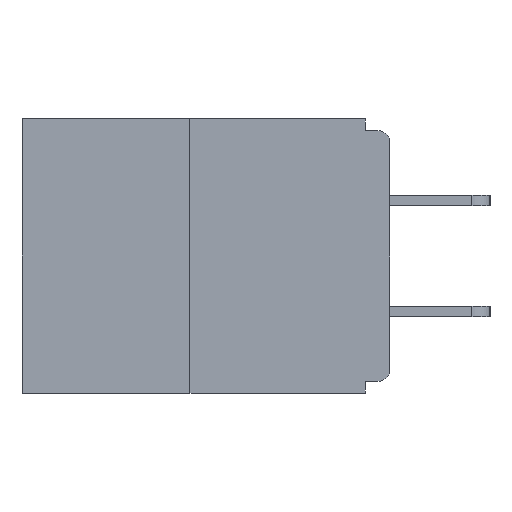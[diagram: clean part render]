
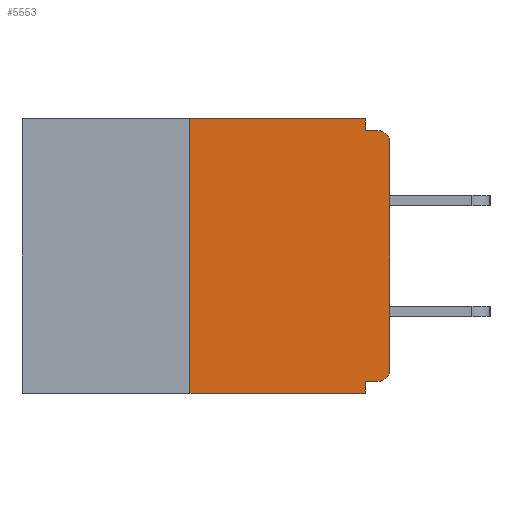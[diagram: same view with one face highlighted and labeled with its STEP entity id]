
A CAD part, left-side view. The second image highlights one B-rep face of the part: STEP entity #5553.
In plain terms, the highlighted planar face has unit normal (-1, 0, 0).
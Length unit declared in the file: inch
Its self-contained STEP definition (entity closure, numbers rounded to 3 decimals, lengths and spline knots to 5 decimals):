
#9 = CARTESIAN_POINT ( 'NONE',  ( 0., 0.031, -0.343 ) ) ;
#730 = VERTEX_POINT ( 'NONE', #9 ) ;
#958 = VECTOR ( 'NONE', #14906, 39.37008 ) ;
#1093 = CARTESIAN_POINT ( 'NONE',  ( 0., 0.015, -0.313 ) ) ;
#1109 = DIRECTION ( 'NONE',  ( 0., -1., 0. ) ) ;
#1291 = VERTEX_POINT ( 'NONE', #16873 ) ;
#1511 = ORIENTED_EDGE ( 'NONE', *, *, #15833, .F. ) ;
#1724 = CARTESIAN_POINT ( 'NONE',  ( 0., 0., -0.03 ) ) ;
#1738 = DIRECTION ( 'NONE',  ( 0., 0., 1. ) ) ;
#2179 = DIRECTION ( 'NONE',  ( 0., 0., -1. ) ) ;
#2210 = VERTEX_POINT ( 'NONE', #12790 ) ;
#2309 = ORIENTED_EDGE ( 'NONE', *, *, #11616, .T. ) ;
#2438 = VERTEX_POINT ( 'NONE', #8670 ) ;
#2523 = LINE ( 'NONE', #8160, #10236 ) ;
#2908 = VERTEX_POINT ( 'NONE', #13664 ) ;
#3392 = EDGE_CURVE ( 'NONE', #2210, #2438, #9552, .T. ) ;
#3741 = ORIENTED_EDGE ( 'NONE', *, *, #15880, .F. ) ;
#3826 = CARTESIAN_POINT ( 'NONE',  ( 0., 0.46, 0. ) ) ;
#4283 = VECTOR ( 'NONE', #13212, 39.37008 ) ;
#4458 = VECTOR ( 'NONE', #1109, 39.37008 ) ;
#4940 = DIRECTION ( 'NONE',  ( -1., 0., 0. ) ) ;
#5096 = EDGE_CURVE ( 'NONE', #2210, #730, #12854, .T. ) ;
#5266 = FACE_OUTER_BOUND ( 'NONE', #16111, .T. ) ;
#5387 = ORIENTED_EDGE ( 'NONE', *, *, #9527, .F. ) ;
#5483 = DIRECTION ( 'NONE',  ( -1., 0., 0. ) ) ;
#5553 = ADVANCED_FACE ( 'NONE', ( #5266 ), #6239, .F. ) ;
#5596 = CARTESIAN_POINT ( 'NONE',  ( 0., 0., -0.313 ) ) ;
#5627 = CARTESIAN_POINT ( 'NONE',  ( 0., 0.015, -0.328 ) ) ;
#5734 = DIRECTION ( 'NONE',  ( 0., 0., -1. ) ) ;
#6239 = PLANE ( 'NONE',  #13242 ) ;
#6266 = ORIENTED_EDGE ( 'NONE', *, *, #5096, .T. ) ;
#6749 = EDGE_CURVE ( 'NONE', #7944, #10308, #14584, .T. ) ;
#6759 = CARTESIAN_POINT ( 'NONE',  ( 0., 0.031, -0.343 ) ) ;
#6808 = CARTESIAN_POINT ( 'NONE',  ( 0., 0., 0. ) ) ;
#7686 = DIRECTION ( 'NONE',  ( 0., 0., -1. ) ) ;
#7709 = EDGE_CURVE ( 'NONE', #2438, #2908, #12510, .T. ) ;
#7856 = ORIENTED_EDGE ( 'NONE', *, *, #15034, .F. ) ;
#7944 = VERTEX_POINT ( 'NONE', #5627 ) ;
#8093 = LINE ( 'NONE', #6808, #4283 ) ;
#8160 = CARTESIAN_POINT ( 'NONE',  ( 0., 0., -0.015 ) ) ;
#8259 = VERTEX_POINT ( 'NONE', #15384 ) ;
#8479 = VERTEX_POINT ( 'NONE', #1724 ) ;
#8670 = CARTESIAN_POINT ( 'NONE',  ( 0., 0.25, 0. ) ) ;
#8991 = VECTOR ( 'NONE', #1738, 39.37008 ) ;
#9527 = EDGE_CURVE ( 'NONE', #2908, #1291, #11322, .T. ) ;
#9552 = LINE ( 'NONE', #14761, #8991 ) ;
#10236 = VECTOR ( 'NONE', #16048, 39.37008 ) ;
#10308 = VERTEX_POINT ( 'NONE', #5596 ) ;
#10540 = VECTOR ( 'NONE', #12338, 39.37008 ) ;
#10943 = EDGE_CURVE ( 'NONE', #8479, #13866, #11941, .T. ) ;
#11322 = LINE ( 'NONE', #15162, #10540 ) ;
#11473 = DIRECTION ( 'NONE',  ( 1., 0., 0. ) ) ;
#11534 = CARTESIAN_POINT ( 'NONE',  ( 0., 0.015, -0.015 ) ) ;
#11616 = EDGE_CURVE ( 'NONE', #10308, #8479, #8093, .T. ) ;
#11683 = AXIS2_PLACEMENT_3D ( 'NONE', #13530, #5483, #5734 ) ;
#11807 = CARTESIAN_POINT ( 'NONE',  ( 0., 0., -0.328 ) ) ;
#11893 = DIRECTION ( 'NONE',  ( 0., 0., -1. ) ) ;
#11941 = CIRCLE ( 'NONE', #11683, 0.015 ) ;
#11975 = DIRECTION ( 'NONE',  ( 0., 1., 0. ) ) ;
#12001 = VECTOR ( 'NONE', #11893, 39.37008 ) ;
#12338 = DIRECTION ( 'NONE',  ( 0., 0., -1. ) ) ;
#12340 = ORIENTED_EDGE ( 'NONE', *, *, #7709, .F. ) ;
#12510 = LINE ( 'NONE', #13694, #958 ) ;
#12679 = ORIENTED_EDGE ( 'NONE', *, *, #10943, .T. ) ;
#12790 = CARTESIAN_POINT ( 'NONE',  ( 0., 0.25, -0.343 ) ) ;
#12854 = LINE ( 'NONE', #12929, #4458 ) ;
#12929 = CARTESIAN_POINT ( 'NONE',  ( 0., 0.46, -0.343 ) ) ;
#13212 = DIRECTION ( 'NONE',  ( 0., 0., 1. ) ) ;
#13242 = AXIS2_PLACEMENT_3D ( 'NONE', #3826, #11473, #7686 ) ;
#13530 = CARTESIAN_POINT ( 'NONE',  ( 0., 0.015, -0.03 ) ) ;
#13664 = CARTESIAN_POINT ( 'NONE',  ( 0., 0.031, 0. ) ) ;
#13694 = CARTESIAN_POINT ( 'NONE',  ( 0., 0.46, 0. ) ) ;
#13866 = VERTEX_POINT ( 'NONE', #11534 ) ;
#14333 = ORIENTED_EDGE ( 'NONE', *, *, #6749, .T. ) ;
#14361 = ORIENTED_EDGE ( 'NONE', *, *, #3392, .F. ) ;
#14584 = CIRCLE ( 'NONE', #15702, 0.015 ) ;
#14617 = LINE ( 'NONE', #6759, #12001 ) ;
#14730 = VECTOR ( 'NONE', #11975, 39.37008 ) ;
#14761 = CARTESIAN_POINT ( 'NONE',  ( 0., 0.25, 0. ) ) ;
#14906 = DIRECTION ( 'NONE',  ( 0., -1., 0. ) ) ;
#15034 = EDGE_CURVE ( 'NONE', #1291, #13866, #2523, .T. ) ;
#15162 = CARTESIAN_POINT ( 'NONE',  ( 0., 0.031, 0. ) ) ;
#15384 = CARTESIAN_POINT ( 'NONE',  ( 0., 0.031, -0.328 ) ) ;
#15702 = AXIS2_PLACEMENT_3D ( 'NONE', #1093, #4940, #2179 ) ;
#15833 = EDGE_CURVE ( 'NONE', #8259, #730, #14617, .T. ) ;
#15880 = EDGE_CURVE ( 'NONE', #7944, #8259, #16003, .T. ) ;
#16003 = LINE ( 'NONE', #11807, #14730 ) ;
#16048 = DIRECTION ( 'NONE',  ( 0., -1., 0. ) ) ;
#16111 = EDGE_LOOP ( 'NONE', ( #12340, #14361, #6266, #1511, #3741, #14333, #2309, #12679, #7856, #5387 ) ) ;
#16873 = CARTESIAN_POINT ( 'NONE',  ( 0., 0.031, -0.015 ) ) ;
